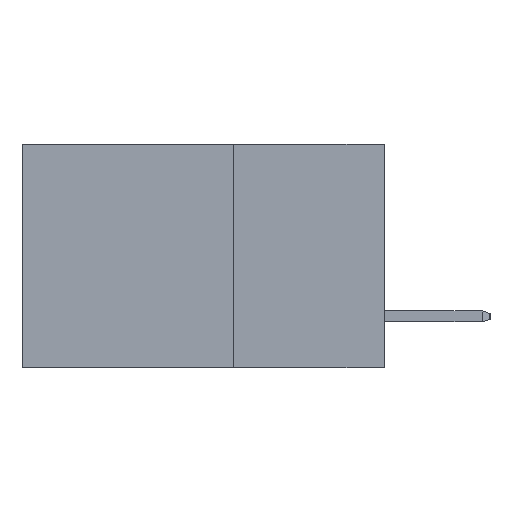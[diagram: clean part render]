
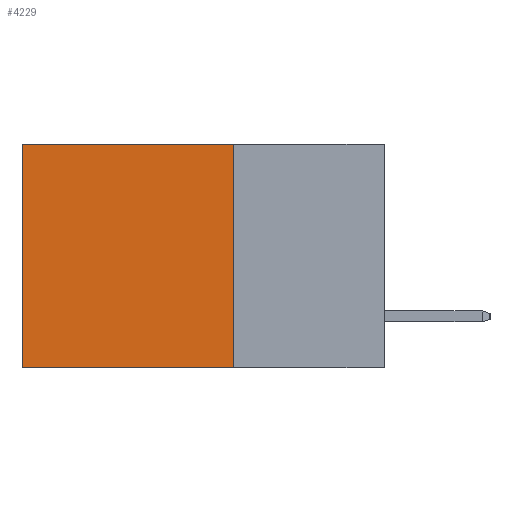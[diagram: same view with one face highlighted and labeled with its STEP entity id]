
A CAD part, left-side view. The second image highlights one B-rep face of the part: STEP entity #4229.
In plain terms, the highlighted planar face has unit normal (-1, 0, 0).
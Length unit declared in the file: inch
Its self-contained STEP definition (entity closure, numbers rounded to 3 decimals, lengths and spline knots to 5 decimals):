
#162 = VECTOR ( 'NONE', #8297, 39.37008 ) ;
#175 = LINE ( 'NONE', #11439, #17596 ) ;
#1056 = LINE ( 'NONE', #15860, #9716 ) ;
#3107 = ORIENTED_EDGE ( 'NONE', *, *, #11034, .T. ) ;
#3167 = EDGE_CURVE ( 'NONE', #6509, #14550, #175, .T. ) ;
#4229 = ADVANCED_FACE ( 'NONE', ( #9810 ), #10565, .F. ) ;
#5527 = DIRECTION ( 'NONE',  ( 0., 0., -1. ) ) ;
#5625 = CARTESIAN_POINT ( 'NONE',  ( 0.2615, 0.25, -0.37 ) ) ;
#6509 = VERTEX_POINT ( 'NONE', #12129 ) ;
#8151 = CARTESIAN_POINT ( 'NONE',  ( 0.2615, 0.6, -0.37 ) ) ;
#8297 = DIRECTION ( 'NONE',  ( 0., 1., 0. ) ) ;
#8407 = CARTESIAN_POINT ( 'NONE',  ( 0.2615, 0.25, 0. ) ) ;
#8574 = VERTEX_POINT ( 'NONE', #12672 ) ;
#9716 = VECTOR ( 'NONE', #15094, 39.37008 ) ;
#9810 = FACE_OUTER_BOUND ( 'NONE', #20419, .T. ) ;
#10194 = DIRECTION ( 'NONE',  ( 0., 0., -1. ) ) ;
#10217 = DIRECTION ( 'NONE',  ( 1., 0., 0. ) ) ;
#10346 = CARTESIAN_POINT ( 'NONE',  ( 0.2615, 0.25, -0.37 ) ) ;
#10565 = PLANE ( 'NONE',  #16832 ) ;
#11034 = EDGE_CURVE ( 'NONE', #16063, #8574, #13782, .T. ) ;
#11272 = EDGE_CURVE ( 'NONE', #16063, #6509, #12976, .T. ) ;
#11334 = DIRECTION ( 'NONE',  ( 0., 1., 0. ) ) ;
#11439 = CARTESIAN_POINT ( 'NONE',  ( 0.2615, 0.25, -0.37 ) ) ;
#12129 = CARTESIAN_POINT ( 'NONE',  ( 0.2615, 0.25, -0.37 ) ) ;
#12672 = CARTESIAN_POINT ( 'NONE',  ( 0.2615, 0.6, 0. ) ) ;
#12976 = LINE ( 'NONE', #5625, #16843 ) ;
#13782 = LINE ( 'NONE', #8407, #162 ) ;
#14517 = ORIENTED_EDGE ( 'NONE', *, *, #3167, .F. ) ;
#14550 = VERTEX_POINT ( 'NONE', #8151 ) ;
#15047 = ORIENTED_EDGE ( 'NONE', *, *, #11272, .F. ) ;
#15094 = DIRECTION ( 'NONE',  ( 0., 0., -1. ) ) ;
#15394 = EDGE_CURVE ( 'NONE', #8574, #14550, #1056, .T. ) ;
#15860 = CARTESIAN_POINT ( 'NONE',  ( 0.2615, 0.6, -0.37 ) ) ;
#16063 = VERTEX_POINT ( 'NONE', #18071 ) ;
#16832 = AXIS2_PLACEMENT_3D ( 'NONE', #10346, #10217, #10194 ) ;
#16843 = VECTOR ( 'NONE', #5527, 39.37008 ) ;
#17596 = VECTOR ( 'NONE', #11334, 39.37008 ) ;
#18071 = CARTESIAN_POINT ( 'NONE',  ( 0.2615, 0.25, 0. ) ) ;
#19898 = ORIENTED_EDGE ( 'NONE', *, *, #15394, .T. ) ;
#20419 = EDGE_LOOP ( 'NONE', ( #19898, #14517, #15047, #3107 ) ) ;
